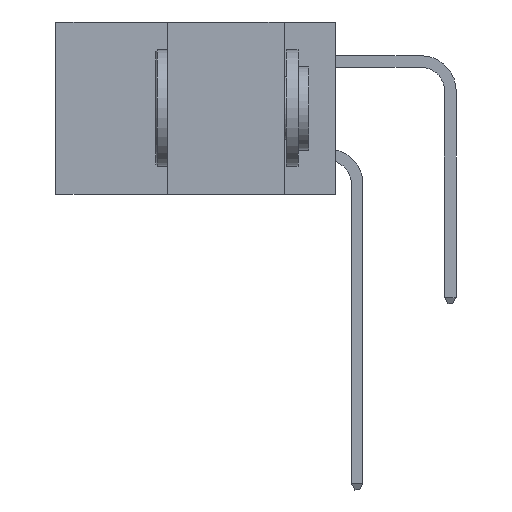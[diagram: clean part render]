
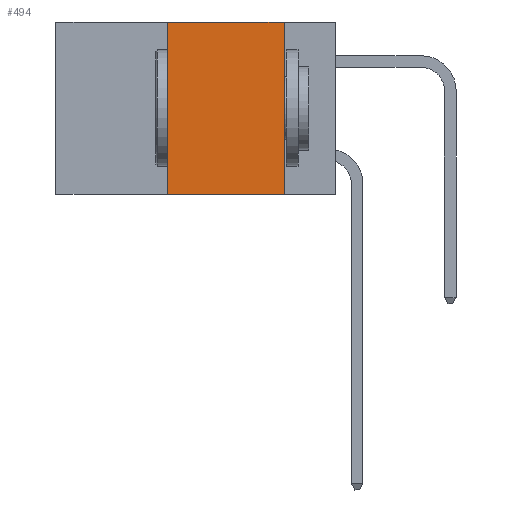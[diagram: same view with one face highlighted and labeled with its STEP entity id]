
A CAD part, left-side view. The second image highlights one B-rep face of the part: STEP entity #494.
In plain terms, the highlighted planar face has unit normal (-1, 0, 0).
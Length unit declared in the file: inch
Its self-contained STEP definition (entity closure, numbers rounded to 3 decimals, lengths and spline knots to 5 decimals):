
#272 = PLANE ( 'NONE',  #13512 ) ;
#494 = ADVANCED_FACE ( 'NONE', ( #10945 ), #272, .F. ) ;
#855 = DIRECTION ( 'NONE',  ( 0., -1., 0. ) ) ;
#1091 = CARTESIAN_POINT ( 'NONE',  ( 0., 0.6, 0. ) ) ;
#1144 = CARTESIAN_POINT ( 'NONE',  ( 0., 0.11, 0. ) ) ;
#1360 = VECTOR ( 'NONE', #855, 39.37008 ) ;
#2646 = EDGE_LOOP ( 'NONE', ( #22774, #27481, #17008, #3178 ) ) ;
#2965 = CARTESIAN_POINT ( 'NONE',  ( 0., 0.6, 0. ) ) ;
#3178 = ORIENTED_EDGE ( 'NONE', *, *, #18527, .T. ) ;
#5512 = CARTESIAN_POINT ( 'NONE',  ( 0., 0.6, -0.37 ) ) ;
#6543 = CARTESIAN_POINT ( 'NONE',  ( 0., 0.11, -0.37 ) ) ;
#7223 = VERTEX_POINT ( 'NONE', #19898 ) ;
#10560 = EDGE_CURVE ( 'NONE', #7223, #21582, #21844, .T. ) ;
#10755 = CARTESIAN_POINT ( 'NONE',  ( 0., 0.36, -0.37 ) ) ;
#10945 = FACE_OUTER_BOUND ( 'NONE', #2646, .T. ) ;
#12318 = CARTESIAN_POINT ( 'NONE',  ( 0., 0.36, 0. ) ) ;
#13497 = EDGE_CURVE ( 'NONE', #21582, #24628, #22042, .T. ) ;
#13512 = AXIS2_PLACEMENT_3D ( 'NONE', #1091, #25248, #26455 ) ;
#14957 = VERTEX_POINT ( 'NONE', #10755 ) ;
#16014 = VECTOR ( 'NONE', #23177, 39.37008 ) ;
#16222 = VECTOR ( 'NONE', #21014, 39.37008 ) ;
#17008 = ORIENTED_EDGE ( 'NONE', *, *, #24363, .F. ) ;
#18527 = EDGE_CURVE ( 'NONE', #14957, #24628, #25168, .T. ) ;
#19898 = CARTESIAN_POINT ( 'NONE',  ( 0., 0.36, 0. ) ) ;
#21014 = DIRECTION ( 'NONE',  ( 0., 0., -1. ) ) ;
#21221 = DIRECTION ( 'NONE',  ( 0., 0., 1. ) ) ;
#21582 = VERTEX_POINT ( 'NONE', #1144 ) ;
#21844 = LINE ( 'NONE', #2965, #16014 ) ;
#22042 = LINE ( 'NONE', #27636, #16222 ) ;
#22774 = ORIENTED_EDGE ( 'NONE', *, *, #13497, .F. ) ;
#23177 = DIRECTION ( 'NONE',  ( 0., -1., 0. ) ) ;
#24363 = EDGE_CURVE ( 'NONE', #14957, #7223, #27816, .T. ) ;
#24628 = VERTEX_POINT ( 'NONE', #6543 ) ;
#25168 = LINE ( 'NONE', #5512, #1360 ) ;
#25248 = DIRECTION ( 'NONE',  ( 1., 0., 0. ) ) ;
#26455 = DIRECTION ( 'NONE',  ( 0., 0., -1. ) ) ;
#27151 = VECTOR ( 'NONE', #21221, 39.37008 ) ;
#27481 = ORIENTED_EDGE ( 'NONE', *, *, #10560, .F. ) ;
#27636 = CARTESIAN_POINT ( 'NONE',  ( 0., 0.11, 0. ) ) ;
#27816 = LINE ( 'NONE', #12318, #27151 ) ;
